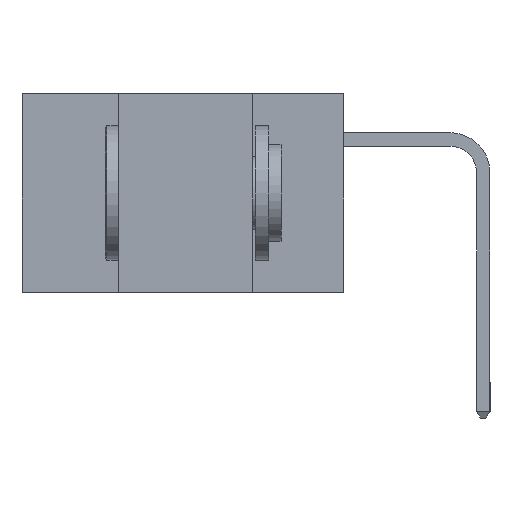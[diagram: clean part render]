
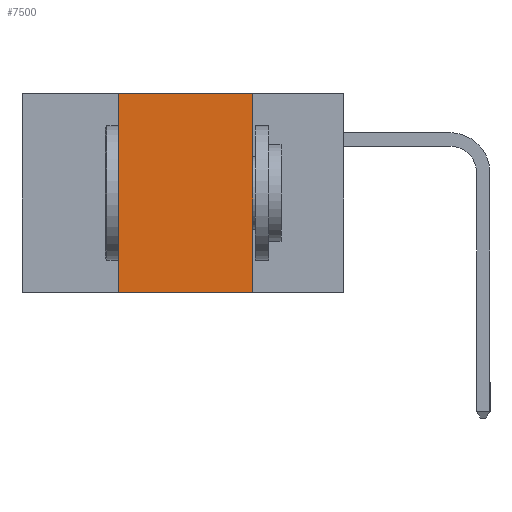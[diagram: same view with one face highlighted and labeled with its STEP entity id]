
A CAD part, left-side view. The second image highlights one B-rep face of the part: STEP entity #7500.
In plain terms, the highlighted planar face has unit normal (-1, 0, 0).
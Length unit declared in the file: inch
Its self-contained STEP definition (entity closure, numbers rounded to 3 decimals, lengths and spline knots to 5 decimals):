
#610 = EDGE_CURVE ( 'NONE', #3295, #11699, #6098, .T. ) ;
#1113 = ORIENTED_EDGE ( 'NONE', *, *, #610, .T. ) ;
#2324 = FACE_OUTER_BOUND ( 'NONE', #10188, .T. ) ;
#3238 = ORIENTED_EDGE ( 'NONE', *, *, #5460, .F. ) ;
#3295 = VERTEX_POINT ( 'NONE', #12614 ) ;
#3437 = DIRECTION ( 'NONE',  ( 0., 0., 1. ) ) ;
#3904 = EDGE_CURVE ( 'NONE', #3295, #13680, #5199, .T. ) ;
#3992 = EDGE_CURVE ( 'NONE', #13680, #10177, #12768, .T. ) ;
#4469 = VECTOR ( 'NONE', #14025, 39.37008 ) ;
#4953 = LINE ( 'NONE', #5531, #7633 ) ;
#5199 = LINE ( 'NONE', #14217, #13835 ) ;
#5279 = DIRECTION ( 'NONE',  ( 0., 0., -1. ) ) ;
#5292 = DIRECTION ( 'NONE',  ( 1., 0., 0. ) ) ;
#5294 = CARTESIAN_POINT ( 'NONE',  ( 0., 0.6, 0. ) ) ;
#5460 = EDGE_CURVE ( 'NONE', #10177, #11699, #4953, .T. ) ;
#5531 = CARTESIAN_POINT ( 'NONE',  ( 0., 0.17, 0. ) ) ;
#6098 = LINE ( 'NONE', #13083, #11759 ) ;
#7244 = PLANE ( 'NONE',  #8176 ) ;
#7500 = ADVANCED_FACE ( 'NONE', ( #2324 ), #7244, .F. ) ;
#7633 = VECTOR ( 'NONE', #8294, 39.37008 ) ;
#7947 = CARTESIAN_POINT ( 'NONE',  ( 0., 0.42, 0. ) ) ;
#8015 = CARTESIAN_POINT ( 'NONE',  ( 0., 0.6, 0. ) ) ;
#8176 = AXIS2_PLACEMENT_3D ( 'NONE', #5294, #5292, #5279 ) ;
#8294 = DIRECTION ( 'NONE',  ( 0., 0., -1. ) ) ;
#9515 = CARTESIAN_POINT ( 'NONE',  ( 0., 0.17, 0. ) ) ;
#9782 = ORIENTED_EDGE ( 'NONE', *, *, #3992, .F. ) ;
#10177 = VERTEX_POINT ( 'NONE', #9515 ) ;
#10188 = EDGE_LOOP ( 'NONE', ( #3238, #9782, #14208, #1113 ) ) ;
#11699 = VERTEX_POINT ( 'NONE', #14778 ) ;
#11759 = VECTOR ( 'NONE', #13581, 39.37008 ) ;
#12614 = CARTESIAN_POINT ( 'NONE',  ( 0., 0.42, -0.37 ) ) ;
#12768 = LINE ( 'NONE', #8015, #4469 ) ;
#13083 = CARTESIAN_POINT ( 'NONE',  ( 0., 0.6, -0.37 ) ) ;
#13581 = DIRECTION ( 'NONE',  ( 0., -1., 0. ) ) ;
#13680 = VERTEX_POINT ( 'NONE', #7947 ) ;
#13835 = VECTOR ( 'NONE', #3437, 39.37008 ) ;
#14025 = DIRECTION ( 'NONE',  ( 0., -1., 0. ) ) ;
#14208 = ORIENTED_EDGE ( 'NONE', *, *, #3904, .F. ) ;
#14217 = CARTESIAN_POINT ( 'NONE',  ( 0., 0.42, 0. ) ) ;
#14778 = CARTESIAN_POINT ( 'NONE',  ( 0., 0.17, -0.37 ) ) ;
